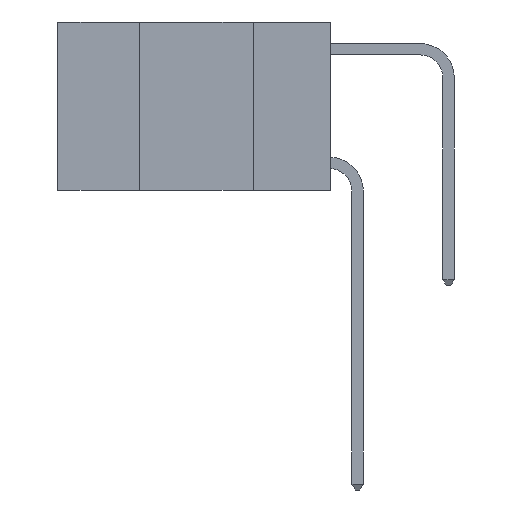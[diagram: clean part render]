
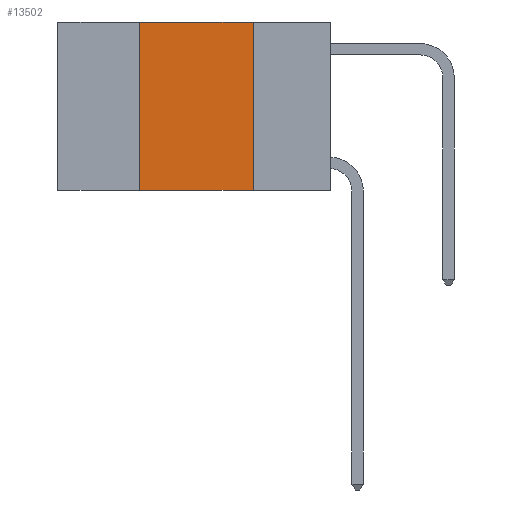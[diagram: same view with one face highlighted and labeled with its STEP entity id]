
A CAD part, left-side view. The second image highlights one B-rep face of the part: STEP entity #13502.
In plain terms, the highlighted planar face has unit normal (-1, 0, 0).
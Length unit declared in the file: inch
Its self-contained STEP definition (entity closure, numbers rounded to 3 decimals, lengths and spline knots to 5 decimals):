
#760 = CARTESIAN_POINT ( 'NONE',  ( 0., 0.17, 0. ) ) ;
#1188 = DIRECTION ( 'NONE',  ( 1., 0., 0. ) ) ;
#1272 = DIRECTION ( 'NONE',  ( 0., 0., 1. ) ) ;
#1294 = DIRECTION ( 'NONE',  ( 0., 0., -1. ) ) ;
#1595 = EDGE_LOOP ( 'NONE', ( #7623, #7275, #6480, #5942 ) ) ;
#2470 = LINE ( 'NONE', #8565, #4638 ) ;
#3081 = VERTEX_POINT ( 'NONE', #10257 ) ;
#3229 = CARTESIAN_POINT ( 'NONE',  ( 0., 0.42, 0. ) ) ;
#3370 = EDGE_CURVE ( 'NONE', #11751, #4135, #8502, .T. ) ;
#4135 = VERTEX_POINT ( 'NONE', #3229 ) ;
#4638 = VECTOR ( 'NONE', #7501, 39.37008 ) ;
#4778 = EDGE_CURVE ( 'NONE', #11033, #3081, #5850, .T. ) ;
#5257 = LINE ( 'NONE', #12695, #7721 ) ;
#5386 = DIRECTION ( 'NONE',  ( 0., -1., 0. ) ) ;
#5505 = CARTESIAN_POINT ( 'NONE',  ( 0., 0.42, 0. ) ) ;
#5528 = CARTESIAN_POINT ( 'NONE',  ( 0., 0.17, 0. ) ) ;
#5850 = LINE ( 'NONE', #5528, #13545 ) ;
#5942 = ORIENTED_EDGE ( 'NONE', *, *, #7602, .T. ) ;
#6480 = ORIENTED_EDGE ( 'NONE', *, *, #3370, .F. ) ;
#7275 = ORIENTED_EDGE ( 'NONE', *, *, #9383, .F. ) ;
#7501 = DIRECTION ( 'NONE',  ( 0., -1., 0. ) ) ;
#7533 = PLANE ( 'NONE',  #9822 ) ;
#7602 = EDGE_CURVE ( 'NONE', #11751, #3081, #2470, .T. ) ;
#7623 = ORIENTED_EDGE ( 'NONE', *, *, #4778, .F. ) ;
#7721 = VECTOR ( 'NONE', #5386, 39.37008 ) ;
#8502 = LINE ( 'NONE', #5505, #10951 ) ;
#8565 = CARTESIAN_POINT ( 'NONE',  ( 0., 0.6, -0.37 ) ) ;
#8607 = DIRECTION ( 'NONE',  ( 0., 0., -1. ) ) ;
#9383 = EDGE_CURVE ( 'NONE', #4135, #11033, #5257, .T. ) ;
#9822 = AXIS2_PLACEMENT_3D ( 'NONE', #12733, #1188, #8607 ) ;
#10257 = CARTESIAN_POINT ( 'NONE',  ( 0., 0.17, -0.37 ) ) ;
#10951 = VECTOR ( 'NONE', #1272, 39.37008 ) ;
#11033 = VERTEX_POINT ( 'NONE', #760 ) ;
#11751 = VERTEX_POINT ( 'NONE', #12467 ) ;
#12467 = CARTESIAN_POINT ( 'NONE',  ( 0., 0.42, -0.37 ) ) ;
#12695 = CARTESIAN_POINT ( 'NONE',  ( 0., 0.6, 0. ) ) ;
#12733 = CARTESIAN_POINT ( 'NONE',  ( 0., 0.6, 0. ) ) ;
#13502 = ADVANCED_FACE ( 'NONE', ( #13504 ), #7533, .F. ) ;
#13504 = FACE_OUTER_BOUND ( 'NONE', #1595, .T. ) ;
#13545 = VECTOR ( 'NONE', #1294, 39.37008 ) ;
